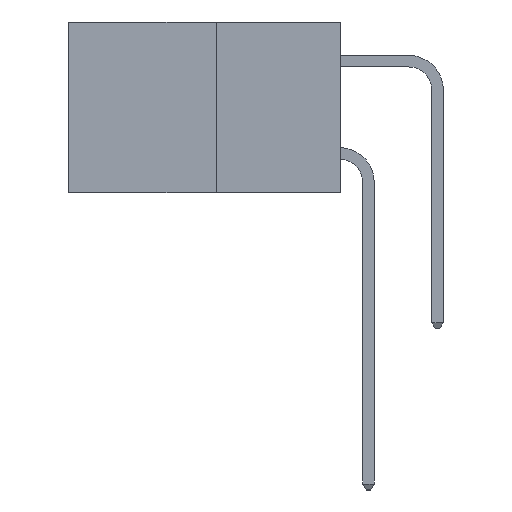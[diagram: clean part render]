
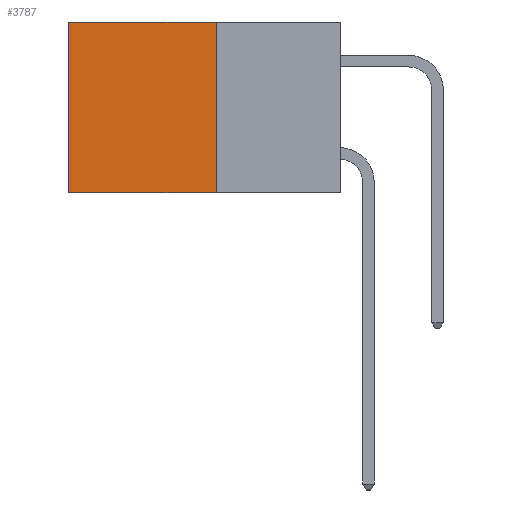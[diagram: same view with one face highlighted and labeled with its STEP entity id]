
A CAD part, left-side view. The second image highlights one B-rep face of the part: STEP entity #3787.
In plain terms, the highlighted planar face has unit normal (-1, 0, 0).
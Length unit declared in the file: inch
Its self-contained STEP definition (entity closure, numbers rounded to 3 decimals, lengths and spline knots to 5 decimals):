
#758 = DIRECTION ( 'NONE',  ( 0., 1., 0. ) ) ;
#1174 = ORIENTED_EDGE ( 'NONE', *, *, #5539, .F. ) ;
#1227 = AXIS2_PLACEMENT_3D ( 'NONE', #10888, #2867, #12194 ) ;
#1229 = VERTEX_POINT ( 'NONE', #2260 ) ;
#1334 = EDGE_CURVE ( 'NONE', #15649, #14656, #13961, .T. ) ;
#1480 = PLANE ( 'NONE',  #1227 ) ;
#2260 = CARTESIAN_POINT ( 'NONE',  ( 0.277, 0.59, 0. ) ) ;
#2401 = EDGE_CURVE ( 'NONE', #1229, #15858, #10593, .T. ) ;
#2867 = DIRECTION ( 'NONE',  ( 1., 0., 0. ) ) ;
#3015 = DIRECTION ( 'NONE',  ( 0., 0., -1. ) ) ;
#3049 = VECTOR ( 'NONE', #3015, 39.37008 ) ;
#3208 = CARTESIAN_POINT ( 'NONE',  ( 0.277, 0.59, -0.37 ) ) ;
#3787 = ADVANCED_FACE ( 'NONE', ( #12331 ), #1480, .F. ) ;
#4188 = ORIENTED_EDGE ( 'NONE', *, *, #8241, .T. ) ;
#4304 = CARTESIAN_POINT ( 'NONE',  ( 0.277, 0.27, -0.37 ) ) ;
#5456 = DIRECTION ( 'NONE',  ( 0., 1., 0. ) ) ;
#5539 = EDGE_CURVE ( 'NONE', #14656, #15858, #10255, .T. ) ;
#5635 = ORIENTED_EDGE ( 'NONE', *, *, #1334, .F. ) ;
#7178 = DIRECTION ( 'NONE',  ( 0., 0., -1. ) ) ;
#8241 = EDGE_CURVE ( 'NONE', #15649, #1229, #15755, .T. ) ;
#8688 = CARTESIAN_POINT ( 'NONE',  ( 0.277, 0.27, -0.37 ) ) ;
#10204 = CARTESIAN_POINT ( 'NONE',  ( 0.277, 0.27, -0.37 ) ) ;
#10255 = LINE ( 'NONE', #10204, #16987 ) ;
#10593 = LINE ( 'NONE', #3208, #3049 ) ;
#10888 = CARTESIAN_POINT ( 'NONE',  ( 0.277, 0.27, -0.37 ) ) ;
#11844 = CARTESIAN_POINT ( 'NONE',  ( 0.277, 0.27, 0. ) ) ;
#12194 = DIRECTION ( 'NONE',  ( 0., 0., -1. ) ) ;
#12331 = FACE_OUTER_BOUND ( 'NONE', #15450, .T. ) ;
#13961 = LINE ( 'NONE', #4304, #14372 ) ;
#14372 = VECTOR ( 'NONE', #7178, 39.37008 ) ;
#14656 = VERTEX_POINT ( 'NONE', #8688 ) ;
#15362 = VECTOR ( 'NONE', #5456, 39.37008 ) ;
#15450 = EDGE_LOOP ( 'NONE', ( #16091, #1174, #5635, #4188 ) ) ;
#15649 = VERTEX_POINT ( 'NONE', #11844 ) ;
#15755 = LINE ( 'NONE', #15897, #15362 ) ;
#15858 = VERTEX_POINT ( 'NONE', #15899 ) ;
#15897 = CARTESIAN_POINT ( 'NONE',  ( 0.277, 0.27, 0. ) ) ;
#15899 = CARTESIAN_POINT ( 'NONE',  ( 0.277, 0.59, -0.37 ) ) ;
#16091 = ORIENTED_EDGE ( 'NONE', *, *, #2401, .T. ) ;
#16987 = VECTOR ( 'NONE', #758, 39.37008 ) ;
